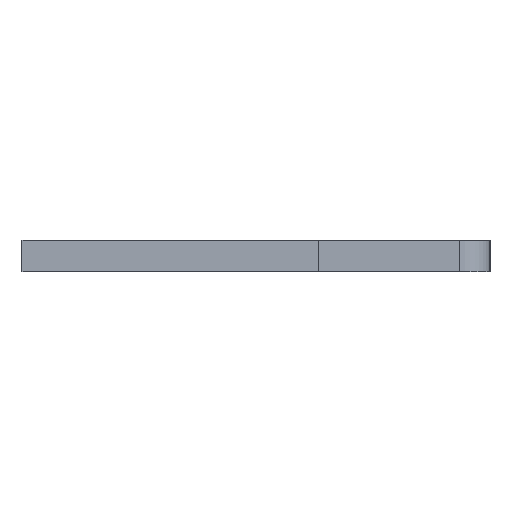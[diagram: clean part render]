
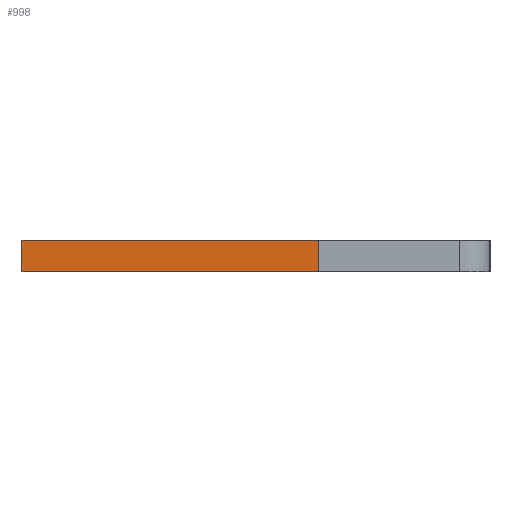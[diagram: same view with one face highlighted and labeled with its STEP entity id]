
A CAD part, left-side view. The second image highlights one B-rep face of the part: STEP entity #998.
In plain terms, the highlighted face is planar.
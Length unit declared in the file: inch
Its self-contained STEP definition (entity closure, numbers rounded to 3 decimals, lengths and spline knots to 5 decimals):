
#17 = LINE ( 'NONE', #2135, #1374 ) ;
#49 = CARTESIAN_POINT ( 'NONE',  ( 0.01, 0.15, -0.04 ) ) ;
#299 = EDGE_LOOP ( 'NONE', ( #2229, #1097, #1902, #545 ) ) ;
#454 = DIRECTION ( 'NONE',  ( 1., 0., 0. ) ) ;
#471 = CARTESIAN_POINT ( 'NONE',  ( 0.01, -0.04, -0.04 ) ) ;
#472 = AXIS2_PLACEMENT_3D ( 'NONE', #49, #2358, #454 ) ;
#513 = LINE ( 'NONE', #1099, #2138 ) ;
#544 = FACE_OUTER_BOUND ( 'NONE', #299, .T. ) ;
#545 = ORIENTED_EDGE ( 'NONE', *, *, #1312, .T. ) ;
#665 = DIRECTION ( 'NONE',  ( 0., 1., 0. ) ) ;
#670 = DIRECTION ( 'NONE',  ( 0., 1., 0. ) ) ;
#693 = DIRECTION ( 'NONE',  ( -1., 0., 0. ) ) ;
#857 = CARTESIAN_POINT ( 'NONE',  ( 0.01, 0.15, -0.04 ) ) ;
#998 = ADVANCED_FACE ( 'NONE', ( #544 ), #1489, .F. ) ;
#1059 = VERTEX_POINT ( 'NONE', #1736 ) ;
#1067 = VECTOR ( 'NONE', #693, 39.37008 ) ;
#1097 = ORIENTED_EDGE ( 'NONE', *, *, #1295, .F. ) ;
#1099 = CARTESIAN_POINT ( 'NONE',  ( -0.01, 0.15, -0.04 ) ) ;
#1102 = VERTEX_POINT ( 'NONE', #1946 ) ;
#1204 = EDGE_CURVE ( 'NONE', #1059, #1102, #2630, .T. ) ;
#1225 = VERTEX_POINT ( 'NONE', #2548 ) ;
#1295 = EDGE_CURVE ( 'NONE', #1102, #1225, #17, .T. ) ;
#1312 = EDGE_CURVE ( 'NONE', #1059, #2558, #2464, .T. ) ;
#1374 = VECTOR ( 'NONE', #1527, 39.37008 ) ;
#1403 = EDGE_CURVE ( 'NONE', #2558, #1225, #513, .T. ) ;
#1489 = PLANE ( 'NONE',  #472 ) ;
#1527 = DIRECTION ( 'NONE',  ( -1., 0., 0. ) ) ;
#1596 = CARTESIAN_POINT ( 'NONE',  ( -0.01, -0.04, -0.04 ) ) ;
#1736 = CARTESIAN_POINT ( 'NONE',  ( 0.01, -0.04, -0.04 ) ) ;
#1902 = ORIENTED_EDGE ( 'NONE', *, *, #1204, .F. ) ;
#1946 = CARTESIAN_POINT ( 'NONE',  ( 0.01, 0.15, -0.04 ) ) ;
#2135 = CARTESIAN_POINT ( 'NONE',  ( 0.01, 0.15, -0.04 ) ) ;
#2138 = VECTOR ( 'NONE', #665, 39.37008 ) ;
#2229 = ORIENTED_EDGE ( 'NONE', *, *, #1403, .T. ) ;
#2358 = DIRECTION ( 'NONE',  ( 0., 0., 1. ) ) ;
#2464 = LINE ( 'NONE', #471, #1067 ) ;
#2528 = VECTOR ( 'NONE', #670, 39.37008 ) ;
#2548 = CARTESIAN_POINT ( 'NONE',  ( -0.01, 0.15, -0.04 ) ) ;
#2558 = VERTEX_POINT ( 'NONE', #1596 ) ;
#2630 = LINE ( 'NONE', #857, #2528 ) ;
